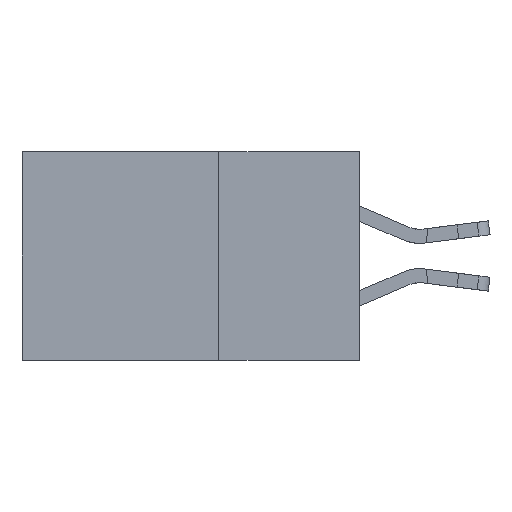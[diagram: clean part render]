
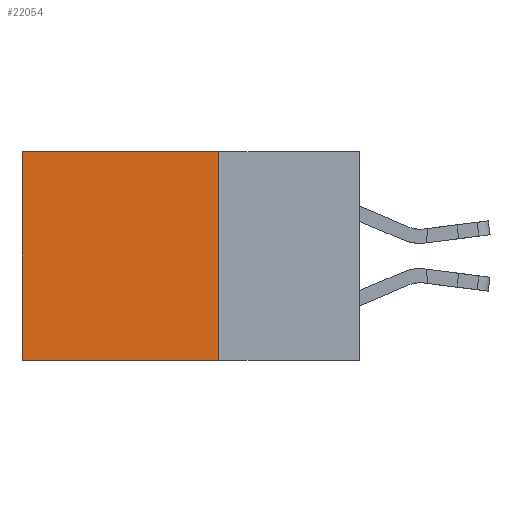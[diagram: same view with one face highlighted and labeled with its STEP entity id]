
A CAD part, left-side view. The second image highlights one B-rep face of the part: STEP entity #22054.
In plain terms, the highlighted planar face has unit normal (-1, 0, 0).
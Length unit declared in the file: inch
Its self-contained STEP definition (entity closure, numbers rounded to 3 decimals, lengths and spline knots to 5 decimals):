
#188 = ORIENTED_EDGE ( 'NONE', *, *, #24255, .T. ) ;
#460 = DIRECTION ( 'NONE',  ( 0., 0., -1. ) ) ;
#547 = FACE_OUTER_BOUND ( 'NONE', #11329, .T. ) ;
#2074 = DIRECTION ( 'NONE',  ( 0., 0., -1. ) ) ;
#3524 = ORIENTED_EDGE ( 'NONE', *, *, #18058, .F. ) ;
#4689 = VERTEX_POINT ( 'NONE', #23595 ) ;
#7735 = CARTESIAN_POINT ( 'NONE',  ( 0.2875, 0.6, -0.37 ) ) ;
#11329 = EDGE_LOOP ( 'NONE', ( #31727, #3524, #16826, #188 ) ) ;
#11953 = CARTESIAN_POINT ( 'NONE',  ( 0.2875, 0.6, 0. ) ) ;
#12971 = CARTESIAN_POINT ( 'NONE',  ( 0.2875, 0.25, 0. ) ) ;
#14560 = LINE ( 'NONE', #12971, #27138 ) ;
#15739 = VECTOR ( 'NONE', #460, 39.37008 ) ;
#15801 = LINE ( 'NONE', #11953, #21702 ) ;
#16826 = ORIENTED_EDGE ( 'NONE', *, *, #19666, .F. ) ;
#17134 = DIRECTION ( 'NONE',  ( 1., 0., 0. ) ) ;
#17188 = DIRECTION ( 'NONE',  ( 0., 1., 0. ) ) ;
#17387 = AXIS2_PLACEMENT_3D ( 'NONE', #32155, #17134, #2074 ) ;
#18058 = EDGE_CURVE ( 'NONE', #4689, #21560, #29595, .T. ) ;
#18758 = EDGE_CURVE ( 'NONE', #26813, #21560, #15801, .T. ) ;
#19666 = EDGE_CURVE ( 'NONE', #30213, #4689, #29882, .T. ) ;
#21560 = VERTEX_POINT ( 'NONE', #7735 ) ;
#21702 = VECTOR ( 'NONE', #27118, 39.37008 ) ;
#22054 = ADVANCED_FACE ( 'NONE', ( #547 ), #27128, .F. ) ;
#22127 = VECTOR ( 'NONE', #17188, 39.37008 ) ;
#23250 = CARTESIAN_POINT ( 'NONE',  ( 0.2875, 0.25, 0. ) ) ;
#23595 = CARTESIAN_POINT ( 'NONE',  ( 0.2875, 0.25, -0.37 ) ) ;
#23754 = CARTESIAN_POINT ( 'NONE',  ( 0.2875, 0.6, 0. ) ) ;
#24255 = EDGE_CURVE ( 'NONE', #30213, #26813, #14560, .T. ) ;
#26813 = VERTEX_POINT ( 'NONE', #23754 ) ;
#27118 = DIRECTION ( 'NONE',  ( 0., 0., -1. ) ) ;
#27128 = PLANE ( 'NONE',  #17387 ) ;
#27138 = VECTOR ( 'NONE', #30533, 39.37008 ) ;
#29595 = LINE ( 'NONE', #32209, #22127 ) ;
#29882 = LINE ( 'NONE', #30591, #15739 ) ;
#30213 = VERTEX_POINT ( 'NONE', #23250 ) ;
#30533 = DIRECTION ( 'NONE',  ( 0., 1., 0. ) ) ;
#30591 = CARTESIAN_POINT ( 'NONE',  ( 0.2875, 0.25, 0. ) ) ;
#31727 = ORIENTED_EDGE ( 'NONE', *, *, #18758, .T. ) ;
#32155 = CARTESIAN_POINT ( 'NONE',  ( 0.2875, 0.25, 0. ) ) ;
#32209 = CARTESIAN_POINT ( 'NONE',  ( 0.2875, 0.25, -0.37 ) ) ;
